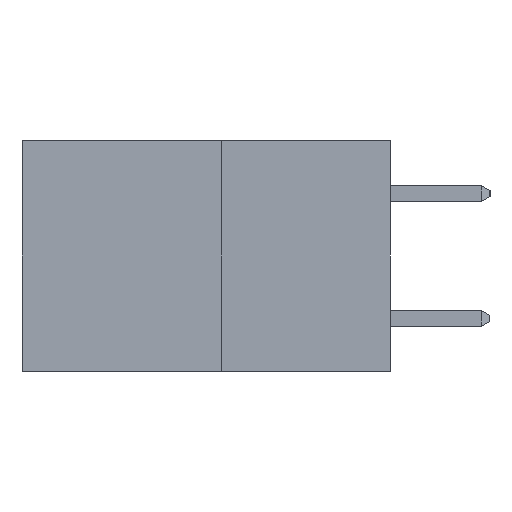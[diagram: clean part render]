
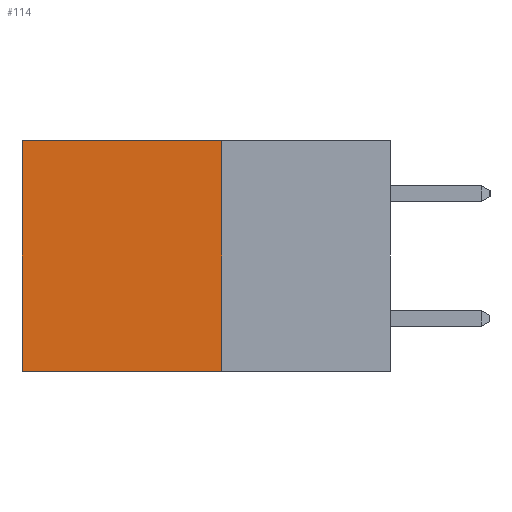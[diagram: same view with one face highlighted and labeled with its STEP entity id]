
A CAD part, left-side view. The second image highlights one B-rep face of the part: STEP entity #114.
In plain terms, the highlighted planar face has unit normal (-1, 0, 0).
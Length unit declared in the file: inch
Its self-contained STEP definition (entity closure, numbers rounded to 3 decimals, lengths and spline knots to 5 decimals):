
#6 = VERTEX_POINT ( 'NONE', #7955 ) ;
#114 = ADVANCED_FACE ( 'NONE', ( #7618 ), #3414, .F. ) ;
#923 = DIRECTION ( 'NONE',  ( 0., 0., -1. ) ) ;
#1358 = CARTESIAN_POINT ( 'NONE',  ( 0.277, 0.27, -0.37 ) ) ;
#1513 = VERTEX_POINT ( 'NONE', #6933 ) ;
#2485 = LINE ( 'NONE', #9557, #7155 ) ;
#2929 = ORIENTED_EDGE ( 'NONE', *, *, #4037, .T. ) ;
#3414 = PLANE ( 'NONE',  #5931 ) ;
#3429 = CARTESIAN_POINT ( 'NONE',  ( 0.277, 0.59, 0. ) ) ;
#3584 = VERTEX_POINT ( 'NONE', #3429 ) ;
#4037 = EDGE_CURVE ( 'NONE', #3584, #5908, #11264, .T. ) ;
#4136 = ORIENTED_EDGE ( 'NONE', *, *, #10047, .F. ) ;
#4279 = DIRECTION ( 'NONE',  ( 1., 0., 0. ) ) ;
#4305 = ORIENTED_EDGE ( 'NONE', *, *, #8191, .F. ) ;
#4363 = DIRECTION ( 'NONE',  ( 0., 0., -1. ) ) ;
#5088 = VECTOR ( 'NONE', #10333, 39.37008 ) ;
#5217 = EDGE_LOOP ( 'NONE', ( #2929, #4136, #4305, #5258 ) ) ;
#5258 = ORIENTED_EDGE ( 'NONE', *, *, #7077, .T. ) ;
#5415 = CARTESIAN_POINT ( 'NONE',  ( 0.277, 0.27, -0.37 ) ) ;
#5429 = LINE ( 'NONE', #9427, #9596 ) ;
#5908 = VERTEX_POINT ( 'NONE', #7536 ) ;
#5931 = AXIS2_PLACEMENT_3D ( 'NONE', #5415, #4279, #4363 ) ;
#6778 = DIRECTION ( 'NONE',  ( 0., 1., 0. ) ) ;
#6933 = CARTESIAN_POINT ( 'NONE',  ( 0.277, 0.27, 0. ) ) ;
#7077 = EDGE_CURVE ( 'NONE', #1513, #3584, #2485, .T. ) ;
#7155 = VECTOR ( 'NONE', #6778, 39.37008 ) ;
#7536 = CARTESIAN_POINT ( 'NONE',  ( 0.277, 0.59, -0.37 ) ) ;
#7543 = LINE ( 'NONE', #1358, #5088 ) ;
#7618 = FACE_OUTER_BOUND ( 'NONE', #5217, .T. ) ;
#7955 = CARTESIAN_POINT ( 'NONE',  ( 0.277, 0.27, -0.37 ) ) ;
#8191 = EDGE_CURVE ( 'NONE', #1513, #6, #7543, .T. ) ;
#9427 = CARTESIAN_POINT ( 'NONE',  ( 0.277, 0.27, -0.37 ) ) ;
#9557 = CARTESIAN_POINT ( 'NONE',  ( 0.277, 0.27, 0. ) ) ;
#9596 = VECTOR ( 'NONE', #10299, 39.37008 ) ;
#10047 = EDGE_CURVE ( 'NONE', #6, #5908, #5429, .T. ) ;
#10299 = DIRECTION ( 'NONE',  ( 0., 1., 0. ) ) ;
#10333 = DIRECTION ( 'NONE',  ( 0., 0., -1. ) ) ;
#10620 = CARTESIAN_POINT ( 'NONE',  ( 0.277, 0.59, -0.37 ) ) ;
#10982 = VECTOR ( 'NONE', #923, 39.37008 ) ;
#11264 = LINE ( 'NONE', #10620, #10982 ) ;
